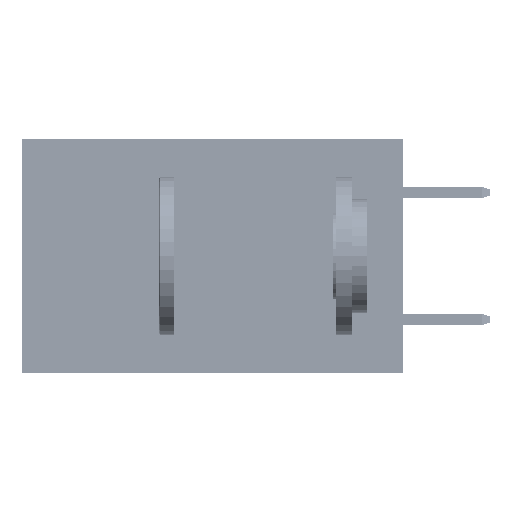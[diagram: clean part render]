
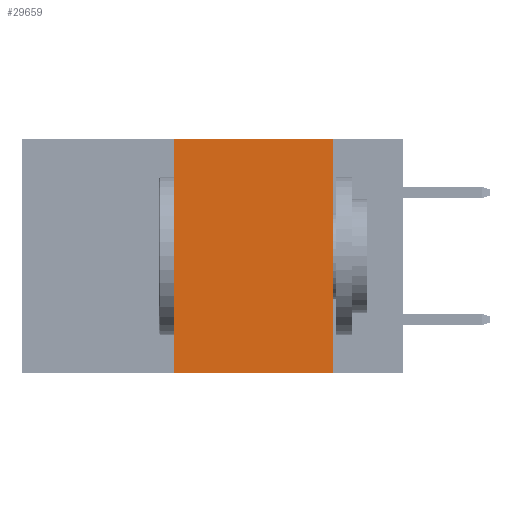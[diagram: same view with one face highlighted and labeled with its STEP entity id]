
A CAD part, left-side view. The second image highlights one B-rep face of the part: STEP entity #29659.
In plain terms, the highlighted planar face has unit normal (-1, 0, 0).
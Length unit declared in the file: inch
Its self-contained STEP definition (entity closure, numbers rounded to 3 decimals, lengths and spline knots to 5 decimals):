
#1684 = LINE ( 'NONE', #14185, #27337 ) ;
#1867 = LINE ( 'NONE', #17760, #31643 ) ;
#1898 = CARTESIAN_POINT ( 'NONE',  ( 0., 0.6, 0. ) ) ;
#2642 = EDGE_CURVE ( 'NONE', #13215, #6707, #1867, .T. ) ;
#6707 = VERTEX_POINT ( 'NONE', #41509 ) ;
#6974 = LINE ( 'NONE', #50923, #19095 ) ;
#10747 = ORIENTED_EDGE ( 'NONE', *, *, #33610, .F. ) ;
#13215 = VERTEX_POINT ( 'NONE', #49709 ) ;
#14185 = CARTESIAN_POINT ( 'NONE',  ( 0., 0.6, -0.37 ) ) ;
#17408 = VERTEX_POINT ( 'NONE', #48948 ) ;
#17760 = CARTESIAN_POINT ( 'NONE',  ( 0., 0.11, 0. ) ) ;
#17789 = DIRECTION ( 'NONE',  ( 1., 0., 0. ) ) ;
#18433 = EDGE_CURVE ( 'NONE', #17408, #6707, #1684, .T. ) ;
#19095 = VECTOR ( 'NONE', #38455, 39.37008 ) ;
#20353 = CARTESIAN_POINT ( 'NONE',  ( 0., 0.36, 0. ) ) ;
#20688 = DIRECTION ( 'NONE',  ( 0., 0., -1. ) ) ;
#24027 = ORIENTED_EDGE ( 'NONE', *, *, #41806, .F. ) ;
#25102 = ORIENTED_EDGE ( 'NONE', *, *, #2642, .F. ) ;
#25651 = DIRECTION ( 'NONE',  ( 0., -1., 0. ) ) ;
#26069 = ORIENTED_EDGE ( 'NONE', *, *, #18433, .T. ) ;
#27337 = VECTOR ( 'NONE', #25651, 39.37008 ) ;
#28664 = LINE ( 'NONE', #44552, #41047 ) ;
#29493 = FACE_OUTER_BOUND ( 'NONE', #46675, .T. ) ;
#29659 = ADVANCED_FACE ( 'NONE', ( #29493 ), #45369, .F. ) ;
#31643 = VECTOR ( 'NONE', #33611, 39.37008 ) ;
#32563 = DIRECTION ( 'NONE',  ( 0., 0., 1. ) ) ;
#33610 = EDGE_CURVE ( 'NONE', #17408, #34892, #28664, .T. ) ;
#33611 = DIRECTION ( 'NONE',  ( 0., 0., -1. ) ) ;
#34892 = VERTEX_POINT ( 'NONE', #20353 ) ;
#38455 = DIRECTION ( 'NONE',  ( 0., -1., 0. ) ) ;
#39528 = AXIS2_PLACEMENT_3D ( 'NONE', #1898, #17789, #20688 ) ;
#41047 = VECTOR ( 'NONE', #32563, 39.37008 ) ;
#41509 = CARTESIAN_POINT ( 'NONE',  ( 0., 0.11, -0.37 ) ) ;
#41806 = EDGE_CURVE ( 'NONE', #34892, #13215, #6974, .T. ) ;
#44552 = CARTESIAN_POINT ( 'NONE',  ( 0., 0.36, 0. ) ) ;
#45369 = PLANE ( 'NONE',  #39528 ) ;
#46675 = EDGE_LOOP ( 'NONE', ( #25102, #24027, #10747, #26069 ) ) ;
#48948 = CARTESIAN_POINT ( 'NONE',  ( 0., 0.36, -0.37 ) ) ;
#49709 = CARTESIAN_POINT ( 'NONE',  ( 0., 0.11, 0. ) ) ;
#50923 = CARTESIAN_POINT ( 'NONE',  ( 0., 0.6, 0. ) ) ;
